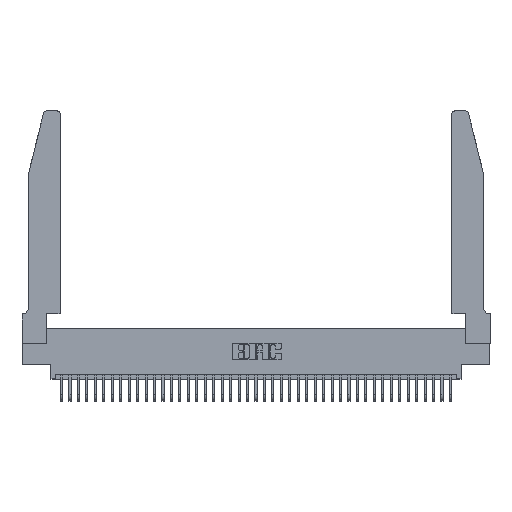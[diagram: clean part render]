
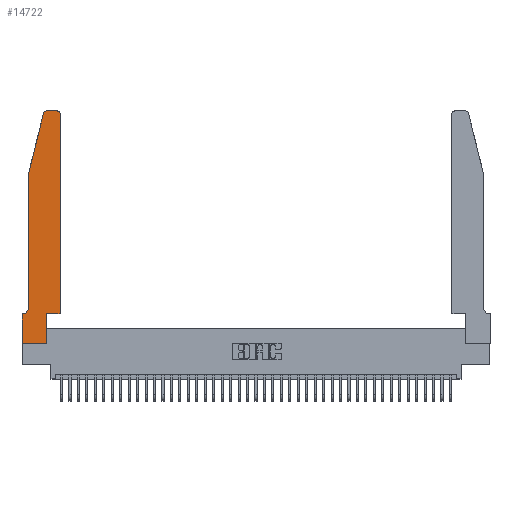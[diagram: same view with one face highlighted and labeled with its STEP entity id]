
A CAD part, top view. The second image highlights one B-rep face of the part: STEP entity #14722.
In plain terms, the highlighted planar face has unit normal (0, 0, 1).
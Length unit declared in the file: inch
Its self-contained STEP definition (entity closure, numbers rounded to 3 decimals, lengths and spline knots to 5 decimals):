
#885 = LINE ( 'NONE', #42600, #20041 ) ;
#978 = DIRECTION ( 'NONE',  ( 0., 1., 0. ) ) ;
#1131 = EDGE_CURVE ( 'NONE', #21894, #41125, #30775, .T. ) ;
#1566 = CARTESIAN_POINT ( 'NONE',  ( 0.0755, 2., 0.37 ) ) ;
#1845 = AXIS2_PLACEMENT_3D ( 'NONE', #24887, #5289, #31880 ) ;
#1859 = ORIENTED_EDGE ( 'NONE', *, *, #7851, .T. ) ;
#2212 = LINE ( 'NONE', #17389, #5280 ) ;
#2238 = VECTOR ( 'NONE', #13303, 39.37008 ) ;
#2309 = VECTOR ( 'NONE', #40988, 39.37008 ) ;
#4018 = VECTOR ( 'NONE', #8613, 39.37008 ) ;
#4444 = EDGE_CURVE ( 'NONE', #24602, #19877, #40371, .T. ) ;
#4690 = AXIS2_PLACEMENT_3D ( 'NONE', #39717, #19978, #10100 ) ;
#4963 = VECTOR ( 'NONE', #978, 39.37008 ) ;
#4964 = DIRECTION ( 'NONE',  ( 0., 0., -1. ) ) ;
#5280 = VECTOR ( 'NONE', #33997, 39.37008 ) ;
#5289 = DIRECTION ( 'NONE',  ( 0., 0., 1. ) ) ;
#5733 = VECTOR ( 'NONE', #23234, 39.37008 ) ;
#5747 = ORIENTED_EDGE ( 'NONE', *, *, #25531, .T. ) ;
#5760 = DIRECTION ( 'NONE',  ( 0., 0., 1. ) ) ;
#5997 = VERTEX_POINT ( 'NONE', #42399 ) ;
#6412 = CARTESIAN_POINT ( 'NONE',  ( 0.0755, 0.35, 0.37 ) ) ;
#6694 = EDGE_CURVE ( 'NONE', #31494, #14684, #15413, .T. ) ;
#7072 = CARTESIAN_POINT ( 'NONE',  ( 0.25487, 2.72718, 0.37 ) ) ;
#7588 = LINE ( 'NONE', #31463, #4018 ) ;
#7851 = EDGE_CURVE ( 'NONE', #13868, #23251, #7588, .T. ) ;
#8613 = DIRECTION ( 'NONE',  ( 0., -1., 0. ) ) ;
#8818 = VERTEX_POINT ( 'NONE', #21308 ) ;
#8883 = PLANE ( 'NONE',  #1845 ) ;
#10100 = DIRECTION ( 'NONE',  ( 1., 0., 0. ) ) ;
#10117 = EDGE_CURVE ( 'NONE', #23251, #24602, #33269, .T. ) ;
#10229 = ORIENTED_EDGE ( 'NONE', *, *, #18843, .T. ) ;
#10554 = EDGE_CURVE ( 'NONE', #27580, #8818, #10991, .T. ) ;
#10684 = DIRECTION ( 'NONE',  ( 0., 1., 0. ) ) ;
#10991 = LINE ( 'NONE', #33002, #2238 ) ;
#11892 = DIRECTION ( 'NONE',  ( 1., 0., 0. ) ) ;
#13303 = DIRECTION ( 'NONE',  ( 1., 0., 0. ) ) ;
#13868 = VERTEX_POINT ( 'NONE', #37712 ) ;
#14083 = CARTESIAN_POINT ( 'NONE',  ( 0.4505, 0.35, 0.37 ) ) ;
#14684 = VERTEX_POINT ( 'NONE', #21101 ) ;
#14722 = ADVANCED_FACE ( 'NONE', ( #16013 ), #8883, .T. ) ;
#15413 = CIRCLE ( 'NONE', #4690, 0.03 ) ;
#15747 = CARTESIAN_POINT ( 'NONE',  ( 0.284, 2.72, 0.37 ) ) ;
#15854 = LINE ( 'NONE', #14083, #4963 ) ;
#16013 = FACE_OUTER_BOUND ( 'NONE', #30763, .T. ) ;
#16685 = ORIENTED_EDGE ( 'NONE', *, *, #10117, .T. ) ;
#17389 = CARTESIAN_POINT ( 'NONE',  ( 0.2605, 2.75, 0.37 ) ) ;
#17807 = LINE ( 'NONE', #1566, #2309 ) ;
#18843 = EDGE_CURVE ( 'NONE', #14684, #5997, #2212, .T. ) ;
#19038 = ORIENTED_EDGE ( 'NONE', *, *, #10554, .T. ) ;
#19382 = CARTESIAN_POINT ( 'NONE',  ( 0., 0., 0.37 ) ) ;
#19507 = CARTESIAN_POINT ( 'NONE',  ( 0.0755, 0.42, 0.37 ) ) ;
#19877 = VERTEX_POINT ( 'NONE', #28486 ) ;
#19978 = DIRECTION ( 'NONE',  ( 0., 0., 1. ) ) ;
#20041 = VECTOR ( 'NONE', #39818, 39.37008 ) ;
#20726 = ORIENTED_EDGE ( 'NONE', *, *, #1131, .T. ) ;
#21068 = DIRECTION ( 'NONE',  ( -1., 0., 0. ) ) ;
#21101 = CARTESIAN_POINT ( 'NONE',  ( 0.4205, 2.75, 0.37 ) ) ;
#21308 = CARTESIAN_POINT ( 'NONE',  ( 0.4505, 0.35, 0.37 ) ) ;
#21894 = VERTEX_POINT ( 'NONE', #19382 ) ;
#21993 = EDGE_CURVE ( 'NONE', #5997, #39681, #32170, .T. ) ;
#22173 = ORIENTED_EDGE ( 'NONE', *, *, #21993, .T. ) ;
#22814 = EDGE_CURVE ( 'NONE', #41125, #27580, #22842, .T. ) ;
#22842 = LINE ( 'NONE', #30640, #25958 ) ;
#23234 = DIRECTION ( 'NONE',  ( -1., 0., 0. ) ) ;
#23251 = VERTEX_POINT ( 'NONE', #19507 ) ;
#24602 = VERTEX_POINT ( 'NONE', #28531 ) ;
#24887 = CARTESIAN_POINT ( 'NONE',  ( 0., 0.35, 0.37 ) ) ;
#25531 = EDGE_CURVE ( 'NONE', #8818, #31494, #15854, .T. ) ;
#25958 = VECTOR ( 'NONE', #10684, 39.37008 ) ;
#27580 = VERTEX_POINT ( 'NONE', #34095 ) ;
#28486 = CARTESIAN_POINT ( 'NONE',  ( 0., 0.35, 0.37 ) ) ;
#28531 = CARTESIAN_POINT ( 'NONE',  ( 0.0055, 0.35, 0.37 ) ) ;
#30482 = AXIS2_PLACEMENT_3D ( 'NONE', #15747, #5760, #32667 ) ;
#30558 = CARTESIAN_POINT ( 'NONE',  ( 0.2865, 0., 0.37 ) ) ;
#30640 = CARTESIAN_POINT ( 'NONE',  ( 0.2865, 0.35, 0.37 ) ) ;
#30763 = EDGE_LOOP ( 'NONE', ( #10229, #22173, #37476, #1859, #16685, #36307, #37204, #20726, #38958, #19038, #5747, #38393 ) ) ;
#30775 = LINE ( 'NONE', #35295, #32882 ) ;
#31463 = CARTESIAN_POINT ( 'NONE',  ( 0.0755, 2., 0.37 ) ) ;
#31494 = VERTEX_POINT ( 'NONE', #38905 ) ;
#31880 = DIRECTION ( 'NONE',  ( 1., 0., 0. ) ) ;
#32170 = CIRCLE ( 'NONE', #30482, 0.03 ) ;
#32667 = DIRECTION ( 'NONE',  ( 1., 0., 0. ) ) ;
#32882 = VECTOR ( 'NONE', #11892, 39.37008 ) ;
#32948 = EDGE_CURVE ( 'NONE', #39681, #13868, #17807, .T. ) ;
#33002 = CARTESIAN_POINT ( 'NONE',  ( 0.4505, 0.35, 0.37 ) ) ;
#33269 = CIRCLE ( 'NONE', #40122, 0.07 ) ;
#33997 = DIRECTION ( 'NONE',  ( -1., 0., 0. ) ) ;
#34095 = CARTESIAN_POINT ( 'NONE',  ( 0.2865, 0.35, 0.37 ) ) ;
#35295 = CARTESIAN_POINT ( 'NONE',  ( 0., 0., 0.37 ) ) ;
#36307 = ORIENTED_EDGE ( 'NONE', *, *, #4444, .T. ) ;
#37204 = ORIENTED_EDGE ( 'NONE', *, *, #42398, .T. ) ;
#37476 = ORIENTED_EDGE ( 'NONE', *, *, #32948, .T. ) ;
#37712 = CARTESIAN_POINT ( 'NONE',  ( 0.0755, 2., 0.37 ) ) ;
#38393 = ORIENTED_EDGE ( 'NONE', *, *, #6694, .T. ) ;
#38905 = CARTESIAN_POINT ( 'NONE',  ( 0.4505, 2.72, 0.37 ) ) ;
#38958 = ORIENTED_EDGE ( 'NONE', *, *, #22814, .T. ) ;
#39681 = VERTEX_POINT ( 'NONE', #7072 ) ;
#39717 = CARTESIAN_POINT ( 'NONE',  ( 0.4205, 2.72, 0.37 ) ) ;
#39818 = DIRECTION ( 'NONE',  ( 0., -1., 0. ) ) ;
#40122 = AXIS2_PLACEMENT_3D ( 'NONE', #41220, #4964, #21068 ) ;
#40371 = LINE ( 'NONE', #6412, #5733 ) ;
#40988 = DIRECTION ( 'NONE',  ( -0.239, -0.971, 0. ) ) ;
#41125 = VERTEX_POINT ( 'NONE', #30558 ) ;
#41220 = CARTESIAN_POINT ( 'NONE',  ( 0.0055, 0.42, 0.37 ) ) ;
#42398 = EDGE_CURVE ( 'NONE', #19877, #21894, #885, .T. ) ;
#42399 = CARTESIAN_POINT ( 'NONE',  ( 0.284, 2.75, 0.37 ) ) ;
#42600 = CARTESIAN_POINT ( 'NONE',  ( 0., 0., 0.37 ) ) ;
